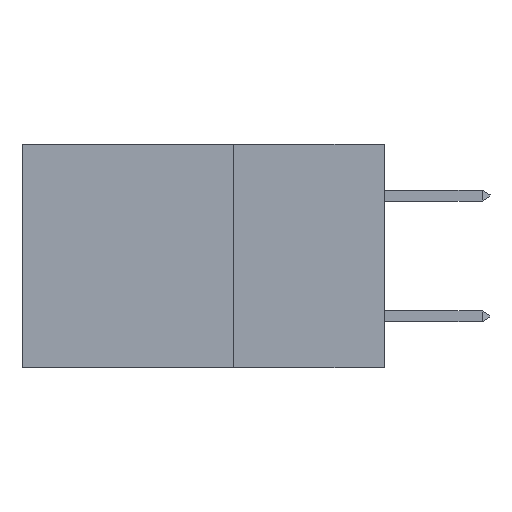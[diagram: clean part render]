
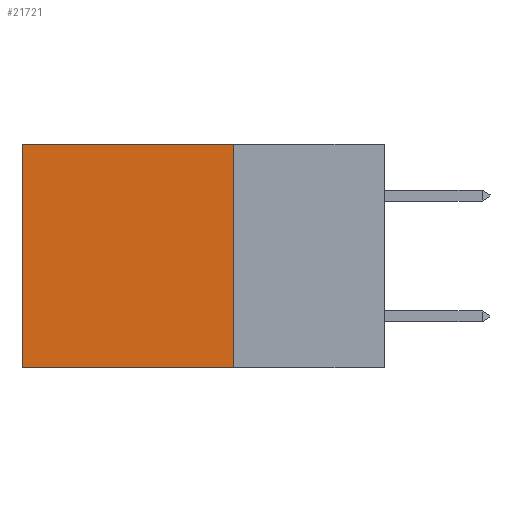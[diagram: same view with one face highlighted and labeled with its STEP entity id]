
A CAD part, left-side view. The second image highlights one B-rep face of the part: STEP entity #21721.
In plain terms, the highlighted planar face has unit normal (-1, 0, 0).
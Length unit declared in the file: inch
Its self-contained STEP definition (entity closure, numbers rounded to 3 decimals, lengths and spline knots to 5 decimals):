
#165 = LINE ( 'NONE', #7667, #10132 ) ;
#812 = DIRECTION ( 'NONE',  ( 0., 1., 0. ) ) ;
#1052 = VERTEX_POINT ( 'NONE', #13052 ) ;
#1247 = DIRECTION ( 'NONE',  ( 0., 0., -1. ) ) ;
#2952 = VERTEX_POINT ( 'NONE', #3468 ) ;
#3337 = CARTESIAN_POINT ( 'NONE',  ( 0.2875, 0.25, 0. ) ) ;
#3468 = CARTESIAN_POINT ( 'NONE',  ( 0.2875, 0.6, -0.37 ) ) ;
#3676 = CARTESIAN_POINT ( 'NONE',  ( 0.2875, 0.25, 0. ) ) ;
#3910 = VERTEX_POINT ( 'NONE', #5307 ) ;
#4035 = EDGE_CURVE ( 'NONE', #1052, #2952, #10883, .T. ) ;
#4690 = VECTOR ( 'NONE', #30174, 39.37008 ) ;
#5307 = CARTESIAN_POINT ( 'NONE',  ( 0.2875, 0.25, -0.37 ) ) ;
#5575 = EDGE_CURVE ( 'NONE', #22212, #1052, #10935, .T. ) ;
#6469 = VECTOR ( 'NONE', #1247, 39.37008 ) ;
#6859 = ORIENTED_EDGE ( 'NONE', *, *, #23698, .F. ) ;
#7667 = CARTESIAN_POINT ( 'NONE',  ( 0.2875, 0.25, -0.37 ) ) ;
#7857 = ORIENTED_EDGE ( 'NONE', *, *, #4035, .T. ) ;
#9159 = DIRECTION ( 'NONE',  ( 0., 0., -1. ) ) ;
#10132 = VECTOR ( 'NONE', #812, 39.37008 ) ;
#10883 = LINE ( 'NONE', #15383, #6469 ) ;
#10935 = LINE ( 'NONE', #18220, #4690 ) ;
#12811 = DIRECTION ( 'NONE',  ( 1., 0., 0. ) ) ;
#13052 = CARTESIAN_POINT ( 'NONE',  ( 0.2875, 0.6, 0. ) ) ;
#13120 = PLANE ( 'NONE',  #13649 ) ;
#13649 = AXIS2_PLACEMENT_3D ( 'NONE', #3337, #12811, #27147 ) ;
#14793 = ORIENTED_EDGE ( 'NONE', *, *, #5575, .T. ) ;
#15383 = CARTESIAN_POINT ( 'NONE',  ( 0.2875, 0.6, 0. ) ) ;
#18070 = ORIENTED_EDGE ( 'NONE', *, *, #27474, .F. ) ;
#18220 = CARTESIAN_POINT ( 'NONE',  ( 0.2875, 0.25, 0. ) ) ;
#18614 = VECTOR ( 'NONE', #9159, 39.37008 ) ;
#19310 = EDGE_LOOP ( 'NONE', ( #7857, #6859, #18070, #14793 ) ) ;
#20799 = CARTESIAN_POINT ( 'NONE',  ( 0.2875, 0.25, 0. ) ) ;
#21721 = ADVANCED_FACE ( 'NONE', ( #29350 ), #13120, .F. ) ;
#22212 = VERTEX_POINT ( 'NONE', #3676 ) ;
#23698 = EDGE_CURVE ( 'NONE', #3910, #2952, #165, .T. ) ;
#27106 = LINE ( 'NONE', #20799, #18614 ) ;
#27147 = DIRECTION ( 'NONE',  ( 0., 0., -1. ) ) ;
#27474 = EDGE_CURVE ( 'NONE', #22212, #3910, #27106, .T. ) ;
#29350 = FACE_OUTER_BOUND ( 'NONE', #19310, .T. ) ;
#30174 = DIRECTION ( 'NONE',  ( 0., 1., 0. ) ) ;
